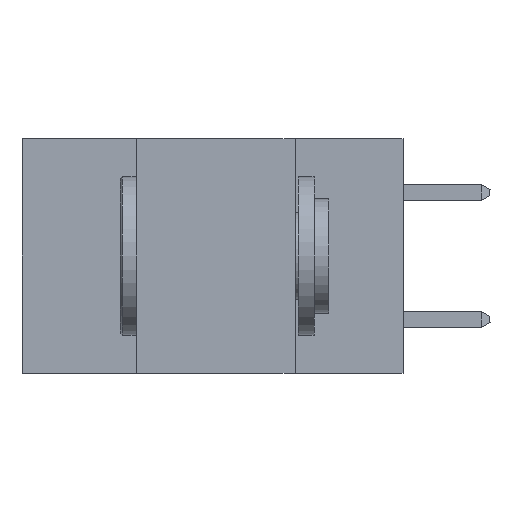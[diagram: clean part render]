
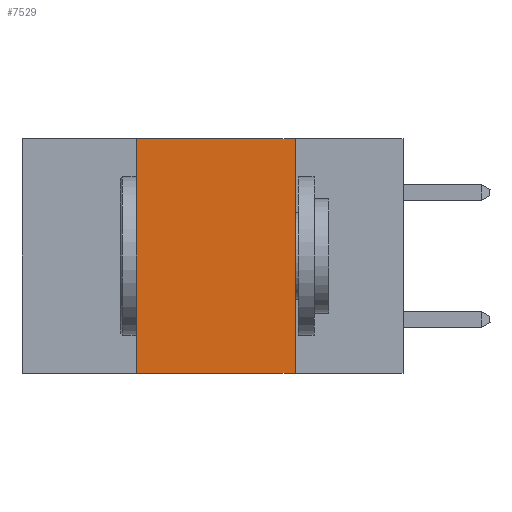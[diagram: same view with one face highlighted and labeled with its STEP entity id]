
A CAD part, left-side view. The second image highlights one B-rep face of the part: STEP entity #7529.
In plain terms, the highlighted planar face has unit normal (-1, 0, 0).
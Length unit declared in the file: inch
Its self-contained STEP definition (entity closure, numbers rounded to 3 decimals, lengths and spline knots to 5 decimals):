
#54 = VERTEX_POINT ( 'NONE', #1142 ) ;
#322 = LINE ( 'NONE', #1640, #5347 ) ;
#798 = DIRECTION ( 'NONE',  ( 0., 0., -1. ) ) ;
#970 = CARTESIAN_POINT ( 'NONE',  ( 0., 0.6, 0. ) ) ;
#1142 = CARTESIAN_POINT ( 'NONE',  ( 0., 0.17, 0. ) ) ;
#1160 = AXIS2_PLACEMENT_3D ( 'NONE', #10340, #8776, #9575 ) ;
#1539 = EDGE_CURVE ( 'NONE', #9821, #2492, #3105, .T. ) ;
#1640 = CARTESIAN_POINT ( 'NONE',  ( 0., 0.42, 0. ) ) ;
#1796 = LINE ( 'NONE', #970, #8834 ) ;
#2172 = CARTESIAN_POINT ( 'NONE',  ( 0., 0.6, -0.37 ) ) ;
#2332 = CARTESIAN_POINT ( 'NONE',  ( 0., 0.42, -0.37 ) ) ;
#2492 = VERTEX_POINT ( 'NONE', #5087 ) ;
#2770 = ORIENTED_EDGE ( 'NONE', *, *, #9282, .F. ) ;
#3105 = LINE ( 'NONE', #2172, #3237 ) ;
#3237 = VECTOR ( 'NONE', #4692, 39.37008 ) ;
#4128 = CARTESIAN_POINT ( 'NONE',  ( 0., 0.42, 0. ) ) ;
#4238 = VECTOR ( 'NONE', #798, 39.37008 ) ;
#4692 = DIRECTION ( 'NONE',  ( 0., -1., 0. ) ) ;
#4825 = CARTESIAN_POINT ( 'NONE',  ( 0., 0.17, 0. ) ) ;
#5087 = CARTESIAN_POINT ( 'NONE',  ( 0., 0.17, -0.37 ) ) ;
#5347 = VECTOR ( 'NONE', #8040, 39.37008 ) ;
#5775 = VERTEX_POINT ( 'NONE', #4128 ) ;
#7210 = PLANE ( 'NONE',  #1160 ) ;
#7518 = EDGE_CURVE ( 'NONE', #54, #2492, #8740, .T. ) ;
#7529 = ADVANCED_FACE ( 'NONE', ( #10373 ), #7210, .F. ) ;
#8040 = DIRECTION ( 'NONE',  ( 0., 0., 1. ) ) ;
#8740 = LINE ( 'NONE', #4825, #4238 ) ;
#8776 = DIRECTION ( 'NONE',  ( 1., 0., 0. ) ) ;
#8834 = VECTOR ( 'NONE', #8939, 39.37008 ) ;
#8939 = DIRECTION ( 'NONE',  ( 0., -1., 0. ) ) ;
#9007 = ORIENTED_EDGE ( 'NONE', *, *, #7518, .F. ) ;
#9117 = EDGE_CURVE ( 'NONE', #9821, #5775, #322, .T. ) ;
#9214 = EDGE_LOOP ( 'NONE', ( #9007, #2770, #10285, #9395 ) ) ;
#9282 = EDGE_CURVE ( 'NONE', #5775, #54, #1796, .T. ) ;
#9395 = ORIENTED_EDGE ( 'NONE', *, *, #1539, .T. ) ;
#9575 = DIRECTION ( 'NONE',  ( 0., 0., -1. ) ) ;
#9821 = VERTEX_POINT ( 'NONE', #2332 ) ;
#10285 = ORIENTED_EDGE ( 'NONE', *, *, #9117, .F. ) ;
#10340 = CARTESIAN_POINT ( 'NONE',  ( 0., 0.6, 0. ) ) ;
#10373 = FACE_OUTER_BOUND ( 'NONE', #9214, .T. ) ;
